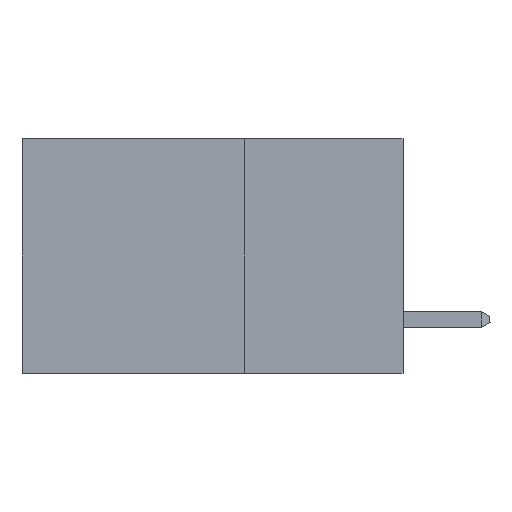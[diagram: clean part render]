
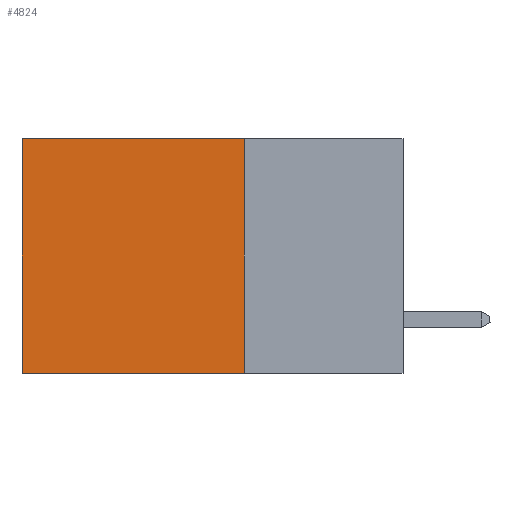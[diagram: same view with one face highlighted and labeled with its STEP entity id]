
A CAD part, left-side view. The second image highlights one B-rep face of the part: STEP entity #4824.
In plain terms, the highlighted planar face has unit normal (-1, 0, 0).
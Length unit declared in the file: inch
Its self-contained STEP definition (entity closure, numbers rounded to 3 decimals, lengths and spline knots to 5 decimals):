
#159 = EDGE_CURVE ( 'NONE', #7452, #3630, #14889, .T. ) ;
#602 = ORIENTED_EDGE ( 'NONE', *, *, #2346, .T. ) ;
#1167 = LINE ( 'NONE', #10871, #9052 ) ;
#1839 = DIRECTION ( 'NONE',  ( 0., 1., 0. ) ) ;
#2346 = EDGE_CURVE ( 'NONE', #15879, #7452, #1167, .T. ) ;
#2428 = DIRECTION ( 'NONE',  ( 1., 0., 0. ) ) ;
#3630 = VERTEX_POINT ( 'NONE', #4066 ) ;
#4054 = CARTESIAN_POINT ( 'NONE',  ( 0.2875, 0.25, 0. ) ) ;
#4066 = CARTESIAN_POINT ( 'NONE',  ( 0.2875, 0.6, -0.37 ) ) ;
#4824 = ADVANCED_FACE ( 'NONE', ( #7335 ), #11594, .F. ) ;
#5507 = CARTESIAN_POINT ( 'NONE',  ( 0.2875, 0.25, 0. ) ) ;
#5633 = VECTOR ( 'NONE', #9642, 39.37008 ) ;
#5967 = CARTESIAN_POINT ( 'NONE',  ( 0.2875, 0.25, -0.37 ) ) ;
#6519 = EDGE_LOOP ( 'NONE', ( #16692, #8572, #11177, #602 ) ) ;
#6923 = CARTESIAN_POINT ( 'NONE',  ( 0.2875, 0.25, -0.37 ) ) ;
#7335 = FACE_OUTER_BOUND ( 'NONE', #6519, .T. ) ;
#7452 = VERTEX_POINT ( 'NONE', #12038 ) ;
#8572 = ORIENTED_EDGE ( 'NONE', *, *, #13335, .F. ) ;
#9052 = VECTOR ( 'NONE', #1839, 39.37008 ) ;
#9115 = DIRECTION ( 'NONE',  ( 0., 1., 0. ) ) ;
#9259 = VERTEX_POINT ( 'NONE', #6923 ) ;
#9642 = DIRECTION ( 'NONE',  ( 0., 0., -1. ) ) ;
#10468 = VECTOR ( 'NONE', #9115, 39.37008 ) ;
#10871 = CARTESIAN_POINT ( 'NONE',  ( 0.2875, 0.25, 0. ) ) ;
#11177 = ORIENTED_EDGE ( 'NONE', *, *, #16375, .F. ) ;
#11594 = PLANE ( 'NONE',  #15528 ) ;
#11961 = DIRECTION ( 'NONE',  ( 0., 0., -1. ) ) ;
#12038 = CARTESIAN_POINT ( 'NONE',  ( 0.2875, 0.6, 0. ) ) ;
#13335 = EDGE_CURVE ( 'NONE', #9259, #3630, #14336, .T. ) ;
#14010 = VECTOR ( 'NONE', #11961, 39.37008 ) ;
#14336 = LINE ( 'NONE', #5967, #10468 ) ;
#14431 = DIRECTION ( 'NONE',  ( 0., 0., -1. ) ) ;
#14889 = LINE ( 'NONE', #14901, #5633 ) ;
#14901 = CARTESIAN_POINT ( 'NONE',  ( 0.2875, 0.6, 0. ) ) ;
#15528 = AXIS2_PLACEMENT_3D ( 'NONE', #4054, #2428, #14431 ) ;
#15879 = VERTEX_POINT ( 'NONE', #18457 ) ;
#16375 = EDGE_CURVE ( 'NONE', #15879, #9259, #18468, .T. ) ;
#16692 = ORIENTED_EDGE ( 'NONE', *, *, #159, .T. ) ;
#18457 = CARTESIAN_POINT ( 'NONE',  ( 0.2875, 0.25, 0. ) ) ;
#18468 = LINE ( 'NONE', #5507, #14010 ) ;
